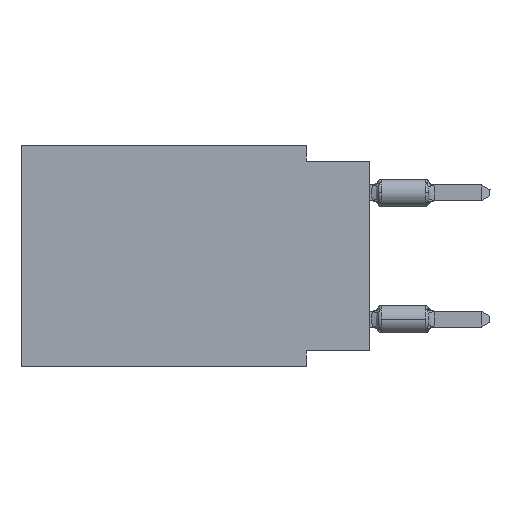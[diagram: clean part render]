
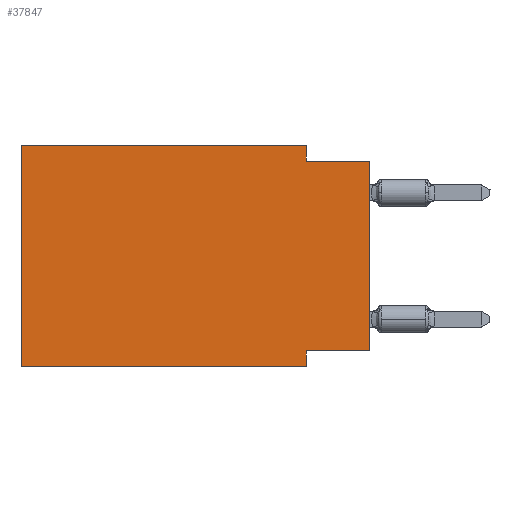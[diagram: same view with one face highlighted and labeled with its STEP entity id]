
A CAD part, left-side view. The second image highlights one B-rep face of the part: STEP entity #37847.
In plain terms, the highlighted planar face has unit normal (-1, 0, 0).
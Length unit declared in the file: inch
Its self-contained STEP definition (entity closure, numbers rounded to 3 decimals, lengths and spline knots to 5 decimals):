
#94 = CARTESIAN_POINT ( 'NONE',  ( 0., 0.1, -0.325 ) ) ;
#833 = LINE ( 'NONE', #4518, #14762 ) ;
#1395 = CARTESIAN_POINT ( 'NONE',  ( 0., 0., -0.025 ) ) ;
#3059 = CARTESIAN_POINT ( 'NONE',  ( 0., 0.1, -0.35 ) ) ;
#3133 = FACE_OUTER_BOUND ( 'NONE', #36093, .T. ) ;
#3331 = DIRECTION ( 'NONE',  ( 0., -1., 0. ) ) ;
#3606 = VERTEX_POINT ( 'NONE', #7380 ) ;
#4518 = CARTESIAN_POINT ( 'NONE',  ( 0., 0., 0. ) ) ;
#6152 = PLANE ( 'NONE',  #8026 ) ;
#6768 = ORIENTED_EDGE ( 'NONE', *, *, #42415, .F. ) ;
#7055 = DIRECTION ( 'NONE',  ( 0., -1., 0. ) ) ;
#7380 = CARTESIAN_POINT ( 'NONE',  ( 0., 0.1, 0. ) ) ;
#8026 = AXIS2_PLACEMENT_3D ( 'NONE', #19379, #32612, #33031 ) ;
#8868 = VERTEX_POINT ( 'NONE', #94 ) ;
#9237 = VERTEX_POINT ( 'NONE', #38634 ) ;
#10087 = EDGE_CURVE ( 'NONE', #14550, #33382, #17846, .T. ) ;
#10994 = CARTESIAN_POINT ( 'NONE',  ( 0., 0.55, 0. ) ) ;
#11220 = LINE ( 'NONE', #10994, #27628 ) ;
#12113 = CARTESIAN_POINT ( 'NONE',  ( 0., 0., -0.325 ) ) ;
#12324 = LINE ( 'NONE', #12113, #25602 ) ;
#12736 = ORIENTED_EDGE ( 'NONE', *, *, #10087, .T. ) ;
#13605 = CARTESIAN_POINT ( 'NONE',  ( 0., 0.1, 0. ) ) ;
#14550 = VERTEX_POINT ( 'NONE', #22275 ) ;
#14762 = VECTOR ( 'NONE', #17297, 39.37008 ) ;
#15051 = VECTOR ( 'NONE', #40623, 39.37008 ) ;
#15998 = DIRECTION ( 'NONE',  ( 0., 1., 0. ) ) ;
#16603 = VECTOR ( 'NONE', #37004, 39.37008 ) ;
#16966 = LINE ( 'NONE', #30626, #19070 ) ;
#17297 = DIRECTION ( 'NONE',  ( 0., 0., 1. ) ) ;
#17846 = LINE ( 'NONE', #20905, #15051 ) ;
#18034 = VECTOR ( 'NONE', #7055, 39.37008 ) ;
#18435 = CARTESIAN_POINT ( 'NONE',  ( 0., 0., -0.025 ) ) ;
#19045 = CARTESIAN_POINT ( 'NONE',  ( 0., 0.1, -0.025 ) ) ;
#19070 = VECTOR ( 'NONE', #3331, 39.37008 ) ;
#19379 = CARTESIAN_POINT ( 'NONE',  ( 0., 0.55, 0. ) ) ;
#20865 = EDGE_CURVE ( 'NONE', #32359, #30699, #40631, .T. ) ;
#20905 = CARTESIAN_POINT ( 'NONE',  ( 0., 0.55, -0.35 ) ) ;
#21200 = VERTEX_POINT ( 'NONE', #42565 ) ;
#22275 = CARTESIAN_POINT ( 'NONE',  ( 0., 0.55, -0.35 ) ) ;
#22834 = ORIENTED_EDGE ( 'NONE', *, *, #23652, .T. ) ;
#23223 = CARTESIAN_POINT ( 'NONE',  ( 0., 0.1, -0.35 ) ) ;
#23456 = ORIENTED_EDGE ( 'NONE', *, *, #20865, .F. ) ;
#23652 = EDGE_CURVE ( 'NONE', #21200, #30699, #833, .T. ) ;
#24007 = LINE ( 'NONE', #13605, #16603 ) ;
#24458 = DIRECTION ( 'NONE',  ( 0., 0., 1. ) ) ;
#25602 = VECTOR ( 'NONE', #15998, 39.37008 ) ;
#26285 = VECTOR ( 'NONE', #29493, 39.37008 ) ;
#26642 = EDGE_CURVE ( 'NONE', #14550, #9237, #11220, .T. ) ;
#27628 = VECTOR ( 'NONE', #24458, 39.37008 ) ;
#29493 = DIRECTION ( 'NONE',  ( 0., 0., -1. ) ) ;
#30038 = ORIENTED_EDGE ( 'NONE', *, *, #42314, .F. ) ;
#30626 = CARTESIAN_POINT ( 'NONE',  ( 0., 0.55, 0. ) ) ;
#30699 = VERTEX_POINT ( 'NONE', #18435 ) ;
#31291 = ORIENTED_EDGE ( 'NONE', *, *, #37904, .F. ) ;
#32359 = VERTEX_POINT ( 'NONE', #19045 ) ;
#32612 = DIRECTION ( 'NONE',  ( 1., 0., 0. ) ) ;
#32752 = LINE ( 'NONE', #3059, #26285 ) ;
#33031 = DIRECTION ( 'NONE',  ( 0., 0., -1. ) ) ;
#33382 = VERTEX_POINT ( 'NONE', #23223 ) ;
#36093 = EDGE_LOOP ( 'NONE', ( #22834, #23456, #6768, #31291, #39820, #12736, #40964, #30038 ) ) ;
#37004 = DIRECTION ( 'NONE',  ( 0., 0., -1. ) ) ;
#37847 = ADVANCED_FACE ( 'NONE', ( #3133 ), #6152, .F. ) ;
#37904 = EDGE_CURVE ( 'NONE', #9237, #3606, #16966, .T. ) ;
#38634 = CARTESIAN_POINT ( 'NONE',  ( 0., 0.55, 0. ) ) ;
#39820 = ORIENTED_EDGE ( 'NONE', *, *, #26642, .F. ) ;
#40623 = DIRECTION ( 'NONE',  ( 0., -1., 0. ) ) ;
#40631 = LINE ( 'NONE', #1395, #18034 ) ;
#40964 = ORIENTED_EDGE ( 'NONE', *, *, #41982, .F. ) ;
#41982 = EDGE_CURVE ( 'NONE', #8868, #33382, #32752, .T. ) ;
#42314 = EDGE_CURVE ( 'NONE', #21200, #8868, #12324, .T. ) ;
#42415 = EDGE_CURVE ( 'NONE', #3606, #32359, #24007, .T. ) ;
#42565 = CARTESIAN_POINT ( 'NONE',  ( 0., 0., -0.325 ) ) ;
